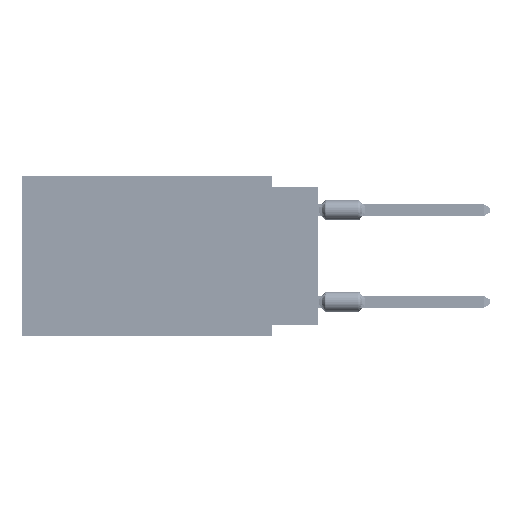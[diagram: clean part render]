
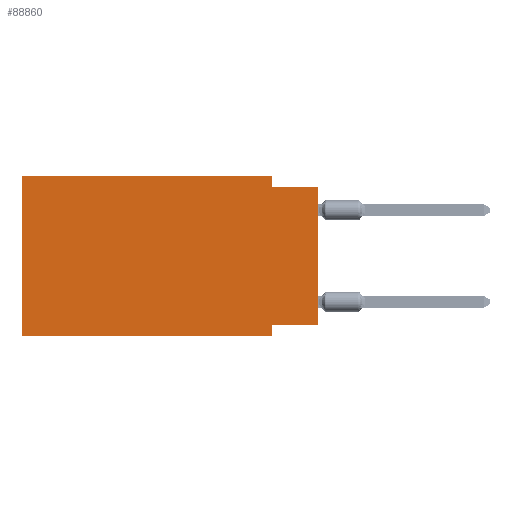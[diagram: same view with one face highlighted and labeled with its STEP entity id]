
A CAD part, left-side view. The second image highlights one B-rep face of the part: STEP entity #88860.
In plain terms, the highlighted planar face has unit normal (-1, 0, 0).
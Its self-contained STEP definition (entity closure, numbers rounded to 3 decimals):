
#2366 = VERTEX_POINT ( 'NONE', #5680 ) ;
#3829 = CARTESIAN_POINT ( 'NONE',  ( 0., 16.383, 0. ) ) ;
#4126 = FACE_OUTER_BOUND ( 'NONE', #59353, .T. ) ;
#4189 = ORIENTED_EDGE ( 'NONE', *, *, #68091, .F. ) ;
#4636 = CARTESIAN_POINT ( 'NONE',  ( 0., 16.383, 0. ) ) ;
#5438 = ORIENTED_EDGE ( 'NONE', *, *, #81843, .F. ) ;
#5680 = CARTESIAN_POINT ( 'NONE',  ( 0., 2.54, -8.89 ) ) ;
#7535 = CARTESIAN_POINT ( 'NONE',  ( 0., 0., -8.255 ) ) ;
#10786 = VECTOR ( 'NONE', #91257, 1000. ) ;
#14654 = LINE ( 'NONE', #7535, #67829 ) ;
#15307 = CARTESIAN_POINT ( 'NONE',  ( 0., 16.383, 0. ) ) ;
#16398 = CARTESIAN_POINT ( 'NONE',  ( 0., 2.54, -8.89 ) ) ;
#16717 = LINE ( 'NONE', #94155, #24067 ) ;
#17550 = DIRECTION ( 'NONE',  ( 0., 0., 1. ) ) ;
#19017 = VECTOR ( 'NONE', #30659, 1000. ) ;
#19477 = EDGE_CURVE ( 'NONE', #99111, #26244, #14654, .T. ) ;
#22564 = LINE ( 'NONE', #30162, #19017 ) ;
#24067 = VECTOR ( 'NONE', #47595, 1000. ) ;
#26244 = VERTEX_POINT ( 'NONE', #56869 ) ;
#27459 = DIRECTION ( 'NONE',  ( 1., 0., 0. ) ) ;
#28369 = VERTEX_POINT ( 'NONE', #32923 ) ;
#29071 = EDGE_CURVE ( 'NONE', #99111, #28369, #66157, .T. ) ;
#30162 = CARTESIAN_POINT ( 'NONE',  ( 0., 0., -0.635 ) ) ;
#30659 = DIRECTION ( 'NONE',  ( 0., -1., 0. ) ) ;
#30849 = DIRECTION ( 'NONE',  ( 0., 1., 0. ) ) ;
#32923 = CARTESIAN_POINT ( 'NONE',  ( 0., 0., -0.635 ) ) ;
#33434 = VECTOR ( 'NONE', #17550, 1000. ) ;
#34072 = ORIENTED_EDGE ( 'NONE', *, *, #66459, .T. ) ;
#35537 = DIRECTION ( 'NONE',  ( 0., 0., -1. ) ) ;
#36133 = VECTOR ( 'NONE', #49248, 1000. ) ;
#37090 = LINE ( 'NONE', #15307, #10786 ) ;
#40697 = VECTOR ( 'NONE', #46748, 1000. ) ;
#40836 = LINE ( 'NONE', #3829, #33434 ) ;
#42492 = VERTEX_POINT ( 'NONE', #82872 ) ;
#46154 = CARTESIAN_POINT ( 'NONE',  ( 0., 16.383, 0. ) ) ;
#46266 = VERTEX_POINT ( 'NONE', #68552 ) ;
#46748 = DIRECTION ( 'NONE',  ( 0., 0., 1. ) ) ;
#47595 = DIRECTION ( 'NONE',  ( 0., 0., -1. ) ) ;
#49248 = DIRECTION ( 'NONE',  ( 0., 0., -1. ) ) ;
#52223 = EDGE_CURVE ( 'NONE', #26244, #2366, #56365, .T. ) ;
#52227 = PLANE ( 'NONE',  #90867 ) ;
#52941 = VECTOR ( 'NONE', #70362, 1000. ) ;
#54763 = ORIENTED_EDGE ( 'NONE', *, *, #52223, .F. ) ;
#56365 = LINE ( 'NONE', #16398, #36133 ) ;
#56869 = CARTESIAN_POINT ( 'NONE',  ( 0., 2.54, -8.255 ) ) ;
#59353 = EDGE_LOOP ( 'NONE', ( #95999, #4189, #74419, #91328, #5438, #34072, #54763, #72209 ) ) ;
#66157 = LINE ( 'NONE', #97030, #40697 ) ;
#66459 = EDGE_CURVE ( 'NONE', #46266, #2366, #90766, .T. ) ;
#67829 = VECTOR ( 'NONE', #30849, 1000. ) ;
#68091 = EDGE_CURVE ( 'NONE', #83412, #28369, #22564, .T. ) ;
#68552 = CARTESIAN_POINT ( 'NONE',  ( 0., 16.383, -8.89 ) ) ;
#70362 = DIRECTION ( 'NONE',  ( 0., -1., 0. ) ) ;
#70627 = CARTESIAN_POINT ( 'NONE',  ( 0., 2.54, -0.635 ) ) ;
#72209 = ORIENTED_EDGE ( 'NONE', *, *, #19477, .F. ) ;
#73237 = EDGE_CURVE ( 'NONE', #42492, #83412, #16717, .T. ) ;
#74419 = ORIENTED_EDGE ( 'NONE', *, *, #73237, .F. ) ;
#78954 = VERTEX_POINT ( 'NONE', #46154 ) ;
#81843 = EDGE_CURVE ( 'NONE', #46266, #78954, #40836, .T. ) ;
#82872 = CARTESIAN_POINT ( 'NONE',  ( 0., 2.54, 0. ) ) ;
#83412 = VERTEX_POINT ( 'NONE', #70627 ) ;
#88032 = CARTESIAN_POINT ( 'NONE',  ( 0., 16.383, -8.89 ) ) ;
#88860 = ADVANCED_FACE ( 'NONE', ( #4126 ), #52227, .F. ) ;
#90766 = LINE ( 'NONE', #88032, #52941 ) ;
#90867 = AXIS2_PLACEMENT_3D ( 'NONE', #4636, #27459, #35537 ) ;
#91257 = DIRECTION ( 'NONE',  ( 0., -1., 0. ) ) ;
#91328 = ORIENTED_EDGE ( 'NONE', *, *, #96232, .F. ) ;
#92339 = CARTESIAN_POINT ( 'NONE',  ( 0., 0., -8.255 ) ) ;
#94155 = CARTESIAN_POINT ( 'NONE',  ( 0., 2.54, 0. ) ) ;
#95999 = ORIENTED_EDGE ( 'NONE', *, *, #29071, .T. ) ;
#96232 = EDGE_CURVE ( 'NONE', #78954, #42492, #37090, .T. ) ;
#97030 = CARTESIAN_POINT ( 'NONE',  ( 0., 0., 0. ) ) ;
#99111 = VERTEX_POINT ( 'NONE', #92339 ) ;
